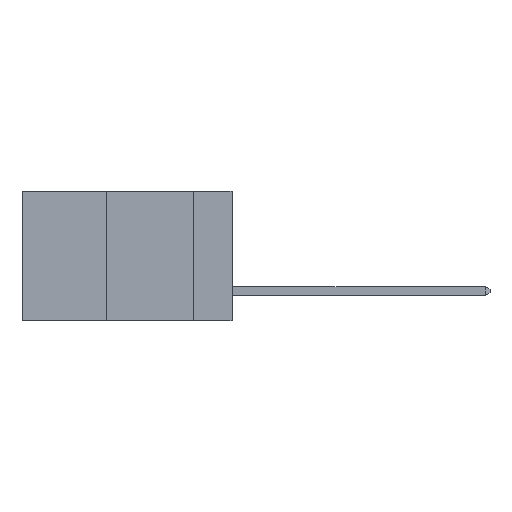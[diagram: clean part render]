
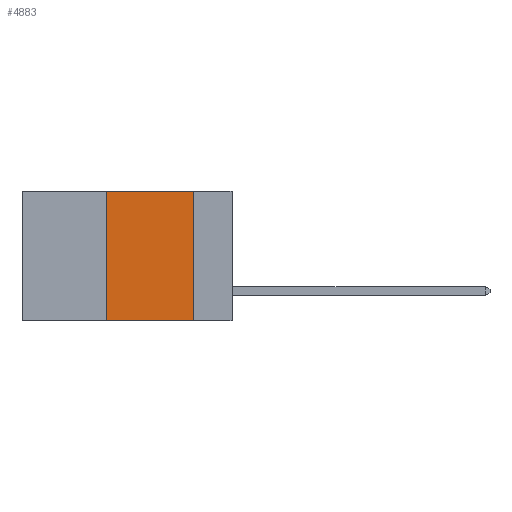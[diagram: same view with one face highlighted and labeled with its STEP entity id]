
A CAD part, left-side view. The second image highlights one B-rep face of the part: STEP entity #4883.
In plain terms, the highlighted planar face has unit normal (-1, 0, 0).
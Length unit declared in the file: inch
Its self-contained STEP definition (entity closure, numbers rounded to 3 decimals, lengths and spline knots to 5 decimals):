
#1269 = VECTOR ( 'NONE', #7696, 39.37008 ) ;
#1790 = ORIENTED_EDGE ( 'NONE', *, *, #19941, .F. ) ;
#2161 = EDGE_LOOP ( 'NONE', ( #9918, #11158, #1790, #22291 ) ) ;
#2237 = FACE_OUTER_BOUND ( 'NONE', #2161, .T. ) ;
#2379 = VECTOR ( 'NONE', #19372, 39.37008 ) ;
#2460 = DIRECTION ( 'NONE',  ( 1., 0., 0. ) ) ;
#2729 = CARTESIAN_POINT ( 'NONE',  ( 0., 0.36, 0. ) ) ;
#2768 = DIRECTION ( 'NONE',  ( 0., 0., 1. ) ) ;
#3613 = VECTOR ( 'NONE', #2768, 39.37008 ) ;
#4230 = AXIS2_PLACEMENT_3D ( 'NONE', #10678, #2460, #4931 ) ;
#4348 = DIRECTION ( 'NONE',  ( 0., 0., -1. ) ) ;
#4362 = VERTEX_POINT ( 'NONE', #12824 ) ;
#4494 = VERTEX_POINT ( 'NONE', #19375 ) ;
#4883 = ADVANCED_FACE ( 'NONE', ( #2237 ), #16509, .F. ) ;
#4931 = DIRECTION ( 'NONE',  ( 0., 0., -1. ) ) ;
#5030 = VECTOR ( 'NONE', #4348, 39.37008 ) ;
#7696 = DIRECTION ( 'NONE',  ( 0., -1., 0. ) ) ;
#9918 = ORIENTED_EDGE ( 'NONE', *, *, #19239, .F. ) ;
#10519 = VERTEX_POINT ( 'NONE', #2729 ) ;
#10678 = CARTESIAN_POINT ( 'NONE',  ( 0., 0.6, 0. ) ) ;
#10987 = EDGE_CURVE ( 'NONE', #16113, #4362, #16134, .T. ) ;
#11158 = ORIENTED_EDGE ( 'NONE', *, *, #14037, .F. ) ;
#11542 = CARTESIAN_POINT ( 'NONE',  ( 0., 0.36, 0. ) ) ;
#12576 = CARTESIAN_POINT ( 'NONE',  ( 0., 0.36, -0.37 ) ) ;
#12824 = CARTESIAN_POINT ( 'NONE',  ( 0., 0.11, -0.37 ) ) ;
#14037 = EDGE_CURVE ( 'NONE', #10519, #4494, #14602, .T. ) ;
#14366 = CARTESIAN_POINT ( 'NONE',  ( 0., 0.6, -0.37 ) ) ;
#14602 = LINE ( 'NONE', #19502, #1269 ) ;
#16113 = VERTEX_POINT ( 'NONE', #12576 ) ;
#16134 = LINE ( 'NONE', #14366, #2379 ) ;
#16509 = PLANE ( 'NONE',  #4230 ) ;
#17836 = LINE ( 'NONE', #11542, #3613 ) ;
#18664 = LINE ( 'NONE', #21321, #5030 ) ;
#19239 = EDGE_CURVE ( 'NONE', #4494, #4362, #18664, .T. ) ;
#19372 = DIRECTION ( 'NONE',  ( 0., -1., 0. ) ) ;
#19375 = CARTESIAN_POINT ( 'NONE',  ( 0., 0.11, 0. ) ) ;
#19502 = CARTESIAN_POINT ( 'NONE',  ( 0., 0.6, 0. ) ) ;
#19941 = EDGE_CURVE ( 'NONE', #16113, #10519, #17836, .T. ) ;
#21321 = CARTESIAN_POINT ( 'NONE',  ( 0., 0.11, 0. ) ) ;
#22291 = ORIENTED_EDGE ( 'NONE', *, *, #10987, .T. ) ;
